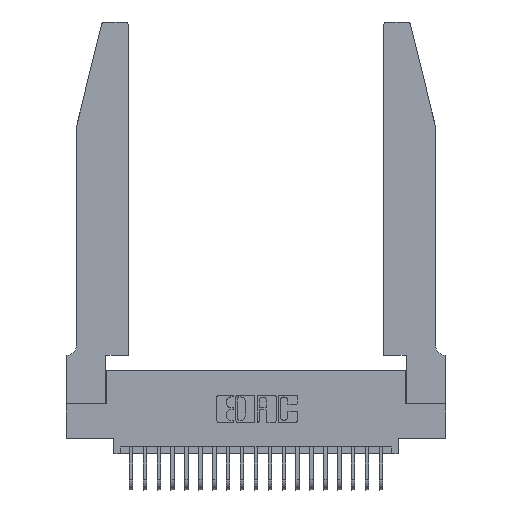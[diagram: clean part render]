
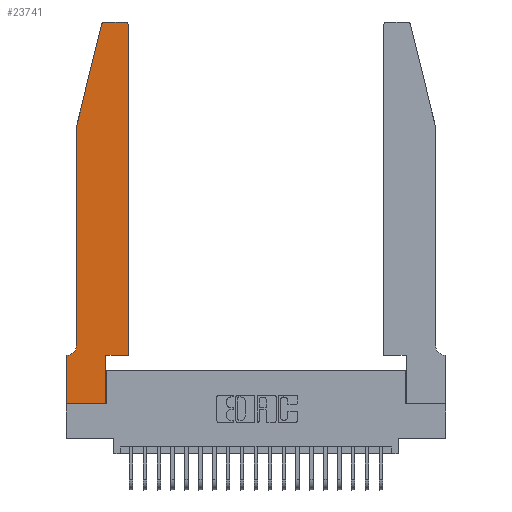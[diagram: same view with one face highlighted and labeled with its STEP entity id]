
A CAD part, top view. The second image highlights one B-rep face of the part: STEP entity #23741.
In plain terms, the highlighted planar face has unit normal (0, 0, 1).
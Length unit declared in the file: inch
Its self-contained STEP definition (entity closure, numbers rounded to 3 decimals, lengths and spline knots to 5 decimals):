
#151 = DIRECTION ( 'NONE',  ( 0., 0., 1. ) ) ;
#270 = VECTOR ( 'NONE', #3969, 39.37008 ) ;
#303 = VERTEX_POINT ( 'NONE', #4654 ) ;
#398 = DIRECTION ( 'NONE',  ( -0.239, -0.971, 0. ) ) ;
#734 = VECTOR ( 'NONE', #9216, 39.37008 ) ;
#764 = EDGE_CURVE ( 'NONE', #1076, #14352, #13970, .T. ) ;
#1063 = EDGE_CURVE ( 'NONE', #7490, #19889, #12464, .T. ) ;
#1076 = VERTEX_POINT ( 'NONE', #17545 ) ;
#1109 = CARTESIAN_POINT ( 'NONE',  ( 0., 0., 0.37 ) ) ;
#1123 = EDGE_CURVE ( 'NONE', #14352, #17412, #11270, .T. ) ;
#1488 = CARTESIAN_POINT ( 'NONE',  ( 0.4505, 0.35, 0.37 ) ) ;
#1644 = DIRECTION ( 'NONE',  ( 0., 1., 0. ) ) ;
#1865 = LINE ( 'NONE', #6592, #6330 ) ;
#2120 = VERTEX_POINT ( 'NONE', #22494 ) ;
#2599 = ORIENTED_EDGE ( 'NONE', *, *, #12830, .T. ) ;
#3147 = AXIS2_PLACEMENT_3D ( 'NONE', #7266, #5428, #18511 ) ;
#3687 = DIRECTION ( 'NONE',  ( 0., 0., 1. ) ) ;
#3969 = DIRECTION ( 'NONE',  ( 1., 0., 0. ) ) ;
#4098 = CARTESIAN_POINT ( 'NONE',  ( 0.0755, 2., 0.37 ) ) ;
#4171 = VECTOR ( 'NONE', #8649, 39.37008 ) ;
#4327 = VERTEX_POINT ( 'NONE', #20063 ) ;
#4368 = ORIENTED_EDGE ( 'NONE', *, *, #1123, .T. ) ;
#4469 = CARTESIAN_POINT ( 'NONE',  ( 0.2865, 0.35, 0.37 ) ) ;
#4632 = EDGE_LOOP ( 'NONE', ( #6470, #9635, #4368, #11444, #17773, #2599, #22865, #6032, #17001, #12746, #11936, #10509 ) ) ;
#4654 = CARTESIAN_POINT ( 'NONE',  ( 0.4205, 2.75, 0.37 ) ) ;
#5428 = DIRECTION ( 'NONE',  ( 0., 0., -1. ) ) ;
#5716 = CARTESIAN_POINT ( 'NONE',  ( 0., 0., 0.37 ) ) ;
#5881 = CARTESIAN_POINT ( 'NONE',  ( 0.4205, 2.72, 0.37 ) ) ;
#6032 = ORIENTED_EDGE ( 'NONE', *, *, #16260, .T. ) ;
#6185 = CARTESIAN_POINT ( 'NONE',  ( 0.25487, 2.72718, 0.37 ) ) ;
#6330 = VECTOR ( 'NONE', #21948, 39.37008 ) ;
#6470 = ORIENTED_EDGE ( 'NONE', *, *, #22409, .T. ) ;
#6592 = CARTESIAN_POINT ( 'NONE',  ( 0.2605, 2.75, 0.37 ) ) ;
#7161 = EDGE_CURVE ( 'NONE', #2120, #7490, #18481, .T. ) ;
#7165 = DIRECTION ( 'NONE',  ( 0., -1., 0. ) ) ;
#7266 = CARTESIAN_POINT ( 'NONE',  ( 0.0055, 0.42, 0.37 ) ) ;
#7328 = AXIS2_PLACEMENT_3D ( 'NONE', #5881, #15550, #11536 ) ;
#7460 = CARTESIAN_POINT ( 'NONE',  ( 0.0055, 0.35, 0.37 ) ) ;
#7480 = DIRECTION ( 'NONE',  ( -1., 0., 0. ) ) ;
#7490 = VERTEX_POINT ( 'NONE', #4469 ) ;
#7784 = AXIS2_PLACEMENT_3D ( 'NONE', #22940, #151, #11630 ) ;
#8143 = VECTOR ( 'NONE', #1644, 39.37008 ) ;
#8167 = LINE ( 'NONE', #1488, #734 ) ;
#8649 = DIRECTION ( 'NONE',  ( 1., 0., 0. ) ) ;
#8732 = CARTESIAN_POINT ( 'NONE',  ( 0.0755, 2., 0.37 ) ) ;
#9216 = DIRECTION ( 'NONE',  ( 0., 1., 0. ) ) ;
#9221 = LINE ( 'NONE', #1109, #4171 ) ;
#9635 = ORIENTED_EDGE ( 'NONE', *, *, #764, .T. ) ;
#9782 = EDGE_CURVE ( 'NONE', #21445, #303, #21009, .T. ) ;
#10257 = VECTOR ( 'NONE', #7480, 39.37008 ) ;
#10436 = EDGE_CURVE ( 'NONE', #4327, #19335, #13052, .T. ) ;
#10509 = ORIENTED_EDGE ( 'NONE', *, *, #9782, .T. ) ;
#10928 = PLANE ( 'NONE',  #24400 ) ;
#11270 = LINE ( 'NONE', #11795, #22491 ) ;
#11444 = ORIENTED_EDGE ( 'NONE', *, *, #24276, .T. ) ;
#11536 = DIRECTION ( 'NONE',  ( 1., 0., 0. ) ) ;
#11630 = DIRECTION ( 'NONE',  ( 1., 0., 0. ) ) ;
#11795 = CARTESIAN_POINT ( 'NONE',  ( 0.0755, 2., 0.37 ) ) ;
#11936 = ORIENTED_EDGE ( 'NONE', *, *, #21247, .T. ) ;
#12210 = CARTESIAN_POINT ( 'NONE',  ( 0.4505, 0.35, 0.37 ) ) ;
#12464 = LINE ( 'NONE', #19031, #270 ) ;
#12746 = ORIENTED_EDGE ( 'NONE', *, *, #1063, .T. ) ;
#12830 = EDGE_CURVE ( 'NONE', #15226, #4327, #23546, .T. ) ;
#13052 = LINE ( 'NONE', #5716, #21280 ) ;
#13294 = VERTEX_POINT ( 'NONE', #23679 ) ;
#13310 = CARTESIAN_POINT ( 'NONE',  ( 0.0755, 0.35, 0.37 ) ) ;
#13970 = CIRCLE ( 'NONE', #7784, 0.03 ) ;
#14352 = VERTEX_POINT ( 'NONE', #6185 ) ;
#15226 = VERTEX_POINT ( 'NONE', #7460 ) ;
#15550 = DIRECTION ( 'NONE',  ( 0., 0., 1. ) ) ;
#16260 = EDGE_CURVE ( 'NONE', #19335, #2120, #9221, .T. ) ;
#16857 = CARTESIAN_POINT ( 'NONE',  ( 0., 0.35, 0.37 ) ) ;
#17001 = ORIENTED_EDGE ( 'NONE', *, *, #7161, .T. ) ;
#17412 = VERTEX_POINT ( 'NONE', #4098 ) ;
#17545 = CARTESIAN_POINT ( 'NONE',  ( 0.284, 2.75, 0.37 ) ) ;
#17773 = ORIENTED_EDGE ( 'NONE', *, *, #23749, .T. ) ;
#18481 = LINE ( 'NONE', #24193, #8143 ) ;
#18511 = DIRECTION ( 'NONE',  ( -1., 0., 0. ) ) ;
#19031 = CARTESIAN_POINT ( 'NONE',  ( 0.4505, 0.35, 0.37 ) ) ;
#19335 = VERTEX_POINT ( 'NONE', #21232 ) ;
#19889 = VERTEX_POINT ( 'NONE', #12210 ) ;
#20063 = CARTESIAN_POINT ( 'NONE',  ( 0., 0.35, 0.37 ) ) ;
#20196 = FACE_OUTER_BOUND ( 'NONE', #4632, .T. ) ;
#21009 = CIRCLE ( 'NONE', #7328, 0.03 ) ;
#21232 = CARTESIAN_POINT ( 'NONE',  ( 0., 0., 0.37 ) ) ;
#21247 = EDGE_CURVE ( 'NONE', #19889, #21445, #8167, .T. ) ;
#21280 = VECTOR ( 'NONE', #23025, 39.37008 ) ;
#21445 = VERTEX_POINT ( 'NONE', #22857 ) ;
#21948 = DIRECTION ( 'NONE',  ( -1., 0., 0. ) ) ;
#21958 = CIRCLE ( 'NONE', #3147, 0.07 ) ;
#22409 = EDGE_CURVE ( 'NONE', #303, #1076, #1865, .T. ) ;
#22491 = VECTOR ( 'NONE', #398, 39.37008 ) ;
#22494 = CARTESIAN_POINT ( 'NONE',  ( 0.2865, 0., 0.37 ) ) ;
#22857 = CARTESIAN_POINT ( 'NONE',  ( 0.4505, 2.72, 0.37 ) ) ;
#22865 = ORIENTED_EDGE ( 'NONE', *, *, #10436, .T. ) ;
#22940 = CARTESIAN_POINT ( 'NONE',  ( 0.284, 2.72, 0.37 ) ) ;
#23025 = DIRECTION ( 'NONE',  ( 0., -1., 0. ) ) ;
#23546 = LINE ( 'NONE', #13310, #10257 ) ;
#23679 = CARTESIAN_POINT ( 'NONE',  ( 0.0755, 0.42, 0.37 ) ) ;
#23741 = ADVANCED_FACE ( 'NONE', ( #20196 ), #10928, .T. ) ;
#23749 = EDGE_CURVE ( 'NONE', #13294, #15226, #21958, .T. ) ;
#24030 = LINE ( 'NONE', #8732, #24325 ) ;
#24193 = CARTESIAN_POINT ( 'NONE',  ( 0.2865, 0.35, 0.37 ) ) ;
#24276 = EDGE_CURVE ( 'NONE', #17412, #13294, #24030, .T. ) ;
#24320 = DIRECTION ( 'NONE',  ( 1., 0., 0. ) ) ;
#24325 = VECTOR ( 'NONE', #7165, 39.37008 ) ;
#24400 = AXIS2_PLACEMENT_3D ( 'NONE', #16857, #3687, #24320 ) ;
